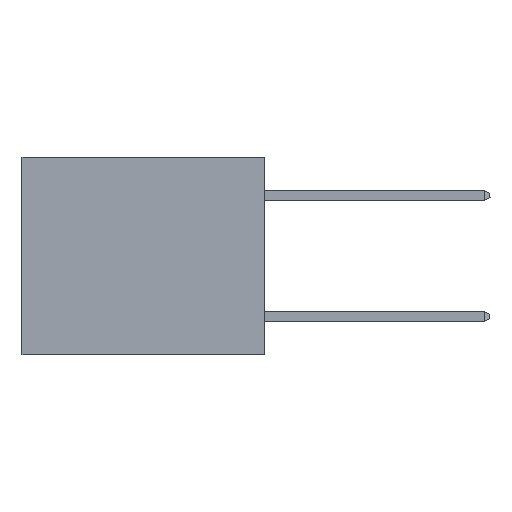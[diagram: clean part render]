
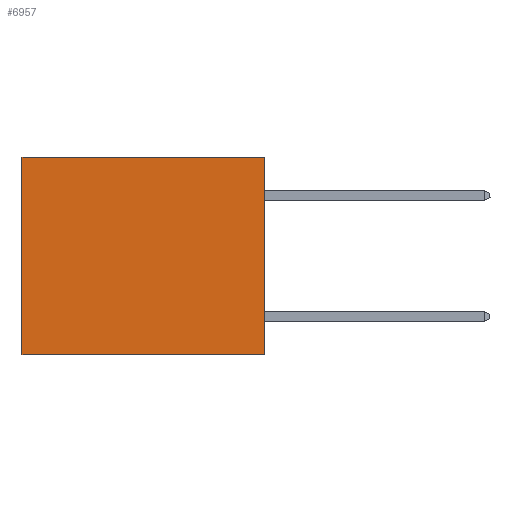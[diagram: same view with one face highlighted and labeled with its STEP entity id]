
A CAD part, left-side view. The second image highlights one B-rep face of the part: STEP entity #6957.
In plain terms, the highlighted planar face has unit normal (-1, 0, 0).
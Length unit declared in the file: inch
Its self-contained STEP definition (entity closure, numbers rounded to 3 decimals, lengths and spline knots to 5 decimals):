
#461 = VECTOR ( 'NONE', #6649, 39.37008 ) ;
#1007 = VERTEX_POINT ( 'NONE', #26077 ) ;
#1196 = LINE ( 'NONE', #22385, #21269 ) ;
#1982 = EDGE_CURVE ( 'NONE', #1007, #17224, #29927, .T. ) ;
#2183 = DIRECTION ( 'NONE',  ( 1., 0., 0. ) ) ;
#2754 = LINE ( 'NONE', #12880, #25801 ) ;
#2993 = VECTOR ( 'NONE', #19104, 39.37008 ) ;
#4937 = VERTEX_POINT ( 'NONE', #26892 ) ;
#5798 = ORIENTED_EDGE ( 'NONE', *, *, #17970, .F. ) ;
#6649 = DIRECTION ( 'NONE',  ( 0., 1., 0. ) ) ;
#6737 = CARTESIAN_POINT ( 'NONE',  ( 0.3165, 0.6, -0.49 ) ) ;
#6957 = ADVANCED_FACE ( 'NONE', ( #17795 ), #28097, .F. ) ;
#7223 = DIRECTION ( 'NONE',  ( 0., 0., -1. ) ) ;
#9241 = LINE ( 'NONE', #6737, #2993 ) ;
#10035 = AXIS2_PLACEMENT_3D ( 'NONE', #28507, #2183, #7223 ) ;
#12593 = ORIENTED_EDGE ( 'NONE', *, *, #12694, .F. ) ;
#12694 = EDGE_CURVE ( 'NONE', #4937, #15817, #2754, .T. ) ;
#12880 = CARTESIAN_POINT ( 'NONE',  ( 0.3165, 0., -0.49 ) ) ;
#15817 = VERTEX_POINT ( 'NONE', #22650 ) ;
#17224 = VERTEX_POINT ( 'NONE', #18248 ) ;
#17634 = DIRECTION ( 'NONE',  ( 0., 1., 0. ) ) ;
#17795 = FACE_OUTER_BOUND ( 'NONE', #29015, .T. ) ;
#17970 = EDGE_CURVE ( 'NONE', #1007, #4937, #1196, .T. ) ;
#18248 = CARTESIAN_POINT ( 'NONE',  ( 0.3165, 0.6, 0. ) ) ;
#19104 = DIRECTION ( 'NONE',  ( 0., 0., -1. ) ) ;
#19771 = DIRECTION ( 'NONE',  ( 0., 0., -1. ) ) ;
#20698 = CARTESIAN_POINT ( 'NONE',  ( 0.3165, 0., 0. ) ) ;
#21269 = VECTOR ( 'NONE', #19771, 39.37008 ) ;
#21727 = ORIENTED_EDGE ( 'NONE', *, *, #30413, .T. ) ;
#22385 = CARTESIAN_POINT ( 'NONE',  ( 0.3165, 0., -0.49 ) ) ;
#22650 = CARTESIAN_POINT ( 'NONE',  ( 0.3165, 0.6, -0.49 ) ) ;
#25801 = VECTOR ( 'NONE', #17634, 39.37008 ) ;
#26077 = CARTESIAN_POINT ( 'NONE',  ( 0.3165, 0., 0. ) ) ;
#26892 = CARTESIAN_POINT ( 'NONE',  ( 0.3165, 0., -0.49 ) ) ;
#28097 = PLANE ( 'NONE',  #10035 ) ;
#28507 = CARTESIAN_POINT ( 'NONE',  ( 0.3165, 0., -0.49 ) ) ;
#29015 = EDGE_LOOP ( 'NONE', ( #21727, #12593, #5798, #30378 ) ) ;
#29927 = LINE ( 'NONE', #20698, #461 ) ;
#30378 = ORIENTED_EDGE ( 'NONE', *, *, #1982, .T. ) ;
#30413 = EDGE_CURVE ( 'NONE', #17224, #15817, #9241, .T. ) ;
